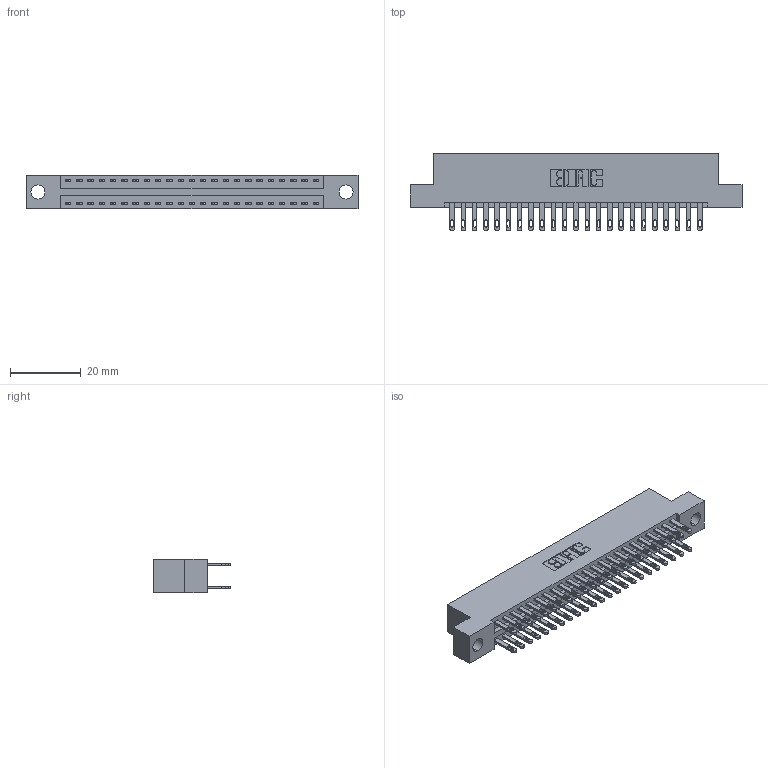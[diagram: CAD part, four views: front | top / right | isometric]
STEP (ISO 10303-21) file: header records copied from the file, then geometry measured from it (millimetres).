
FILE_DESCRIPTION (( 'STEP AP203' ), '1' );
FILE_NAME ('346-046-500-204.STEP', '2022-05-20T08:47:16', ( '' ), ( '' ), 'SwSTEP 2.0', 'SolidWorks 2020', '' );
FILE_SCHEMA (( 'CONFIG_CONTROL_DESIGN' ));
Length unit declared in the file: inch
Products named in the file (3): 346 Part_Flush Mounting Lugs - 0.156 Dia-TH; 346-046-500-204; 345-292-001_345-293-100
Assembly tree (47 placements, depth 2):
  346-046-500-204
    346 Part_Flush Mounting Lugs - 0.156 Dia-TH
    345-292-001_345-293-100  x46
Bounding box: 93.6 x 21.84 x 9.4 mm (x, y, z)
Volume: 9014.1 mm3; surface area: 12421.2 mm2
Topology: 47 solids, 47 shells, 2344 faces, 7127 edges, 4750 vertices
Faces by surface type: plane 1424, cylinder 920
Entity records: 17917 total; most frequent: CARTESIAN_POINT 2982, ORIENTED_EDGE 2914, DIRECTION 2681, EDGE_CURVE 1457, VECTOR 1229, LINE 1229, VERTEX_POINT 970, AXIS2_PLACEMENT_3D 726
